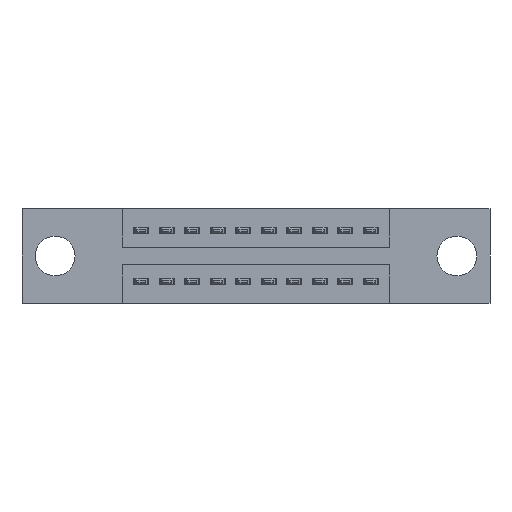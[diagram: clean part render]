
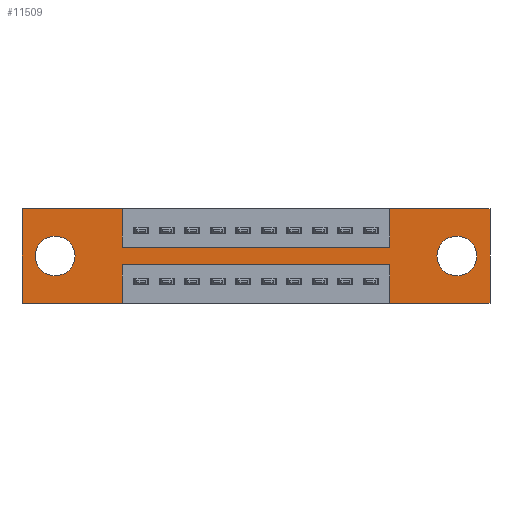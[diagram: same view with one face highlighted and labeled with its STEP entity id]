
A CAD part, front view. The second image highlights one B-rep face of the part: STEP entity #11509.
In plain terms, the highlighted planar face has unit normal (0, -1, 0).
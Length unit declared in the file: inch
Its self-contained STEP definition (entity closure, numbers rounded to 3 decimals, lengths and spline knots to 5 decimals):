
#273 = VERTEX_POINT ( 'NONE', #581 ) ;
#366 = EDGE_LOOP ( 'NONE', ( #4167, #5193, #6597, #5299, #6546, #12338, #12047, #7113, #7534, #8172, #12407, #8401 ) ) ;
#402 = DIRECTION ( 'NONE',  ( 0., 0., 1. ) ) ;
#421 = CIRCLE ( 'NONE', #2617, 0.078 ) ;
#468 = LINE ( 'NONE', #9178, #2892 ) ;
#513 = CARTESIAN_POINT ( 'NONE',  ( 0.3925, 0., -0.22 ) ) ;
#522 = VECTOR ( 'NONE', #561, 39.37008 ) ;
#561 = DIRECTION ( 'NONE',  ( 0., 0., 1. ) ) ;
#581 = CARTESIAN_POINT ( 'NONE',  ( 1.835, 0., 0. ) ) ;
#766 = DIRECTION ( 'NONE',  ( 1., 0., 0. ) ) ;
#969 = CARTESIAN_POINT ( 'NONE',  ( 0.13, 0., -0.107 ) ) ;
#1180 = EDGE_LOOP ( 'NONE', ( #1553, #4073 ) ) ;
#1264 = CARTESIAN_POINT ( 'NONE',  ( 1.835, 0., -0.37 ) ) ;
#1283 = AXIS2_PLACEMENT_3D ( 'NONE', #2928, #3809, #5951 ) ;
#1348 = DIRECTION ( 'NONE',  ( 1., 0., 0. ) ) ;
#1379 = CARTESIAN_POINT ( 'NONE',  ( 0.3925, 0., 0. ) ) ;
#1466 = VERTEX_POINT ( 'NONE', #1264 ) ;
#1487 = DIRECTION ( 'NONE',  ( 0., 0., -1. ) ) ;
#1553 = ORIENTED_EDGE ( 'NONE', *, *, #3692, .T. ) ;
#1842 = VECTOR ( 'NONE', #2558, 39.37008 ) ;
#1938 = FACE_BOUND ( 'NONE', #2115, .T. ) ;
#2027 = CARTESIAN_POINT ( 'NONE',  ( 0.3925, 0., -0.15 ) ) ;
#2050 = EDGE_CURVE ( 'NONE', #2638, #4609, #11177, .T. ) ;
#2115 = EDGE_LOOP ( 'NONE', ( #5553, #5684 ) ) ;
#2297 = CARTESIAN_POINT ( 'NONE',  ( 0., 0., -0.37 ) ) ;
#2338 = VECTOR ( 'NONE', #6648, 39.37008 ) ;
#2358 = DIRECTION ( 'NONE',  ( 0., 0., -1. ) ) ;
#2558 = DIRECTION ( 'NONE',  ( 0., 0., 1. ) ) ;
#2617 = AXIS2_PLACEMENT_3D ( 'NONE', #9967, #3362, #2358 ) ;
#2638 = VERTEX_POINT ( 'NONE', #2777 ) ;
#2651 = EDGE_CURVE ( 'NONE', #273, #1466, #9385, .T. ) ;
#2719 = DIRECTION ( 'NONE',  ( 0., 0., -1. ) ) ;
#2750 = VERTEX_POINT ( 'NONE', #2027 ) ;
#2777 = CARTESIAN_POINT ( 'NONE',  ( 1.4425, 0., -0.22 ) ) ;
#2807 = LINE ( 'NONE', #3710, #2338 ) ;
#2813 = VECTOR ( 'NONE', #9064, 39.37008 ) ;
#2825 = EDGE_CURVE ( 'NONE', #2750, #4581, #8014, .T. ) ;
#2892 = VECTOR ( 'NONE', #7827, 39.37008 ) ;
#2928 = CARTESIAN_POINT ( 'NONE',  ( 0., 0., -0.37 ) ) ;
#2982 = EDGE_CURVE ( 'NONE', #1466, #12223, #2807, .T. ) ;
#3152 = VERTEX_POINT ( 'NONE', #8782 ) ;
#3345 = CARTESIAN_POINT ( 'NONE',  ( 0.13, 0., -0.185 ) ) ;
#3356 = EDGE_CURVE ( 'NONE', #6534, #10361, #7222, .T. ) ;
#3362 = DIRECTION ( 'NONE',  ( 0., 1., 0. ) ) ;
#3375 = VERTEX_POINT ( 'NONE', #6276 ) ;
#3417 = AXIS2_PLACEMENT_3D ( 'NONE', #3345, #11262, #8382 ) ;
#3469 = LINE ( 'NONE', #6373, #8639 ) ;
#3692 = EDGE_CURVE ( 'NONE', #3375, #7938, #421, .T. ) ;
#3710 = CARTESIAN_POINT ( 'NONE',  ( 0., 0., -0.37 ) ) ;
#3809 = DIRECTION ( 'NONE',  ( 0., -1., 0. ) ) ;
#4073 = ORIENTED_EDGE ( 'NONE', *, *, #6514, .T. ) ;
#4167 = ORIENTED_EDGE ( 'NONE', *, *, #8672, .F. ) ;
#4322 = DIRECTION ( 'NONE',  ( -1., 0., 0. ) ) ;
#4442 = AXIS2_PLACEMENT_3D ( 'NONE', #8094, #7005, #1487 ) ;
#4577 = LINE ( 'NONE', #11382, #9696 ) ;
#4581 = VERTEX_POINT ( 'NONE', #10607 ) ;
#4609 = VERTEX_POINT ( 'NONE', #6147 ) ;
#4817 = CARTESIAN_POINT ( 'NONE',  ( 0.3925, 0., -0.37 ) ) ;
#5193 = ORIENTED_EDGE ( 'NONE', *, *, #2050, .F. ) ;
#5299 = ORIENTED_EDGE ( 'NONE', *, *, #2982, .F. ) ;
#5494 = CARTESIAN_POINT ( 'NONE',  ( 1.835, 0., 0. ) ) ;
#5553 = ORIENTED_EDGE ( 'NONE', *, *, #5657, .T. ) ;
#5650 = LINE ( 'NONE', #4817, #7319 ) ;
#5657 = EDGE_CURVE ( 'NONE', #9488, #3152, #8827, .T. ) ;
#5673 = EDGE_CURVE ( 'NONE', #10361, #10035, #8146, .T. ) ;
#5684 = ORIENTED_EDGE ( 'NONE', *, *, #7292, .T. ) ;
#5754 = EDGE_CURVE ( 'NONE', #10035, #2750, #3469, .T. ) ;
#5951 = DIRECTION ( 'NONE',  ( 0., 0., -1. ) ) ;
#5980 = DIRECTION ( 'NONE',  ( 0., 1., 0. ) ) ;
#5991 = CARTESIAN_POINT ( 'NONE',  ( 0.3925, 0., -0.37 ) ) ;
#6147 = CARTESIAN_POINT ( 'NONE',  ( 0.3925, 0., -0.22 ) ) ;
#6276 = CARTESIAN_POINT ( 'NONE',  ( 1.705, 0., -0.107 ) ) ;
#6373 = CARTESIAN_POINT ( 'NONE',  ( 0.3925, 0., 0. ) ) ;
#6387 = CARTESIAN_POINT ( 'NONE',  ( 1.4425, 0., -0.37 ) ) ;
#6472 = CIRCLE ( 'NONE', #9676, 0.078 ) ;
#6489 = CARTESIAN_POINT ( 'NONE',  ( 1.705, 0., -0.263 ) ) ;
#6514 = EDGE_CURVE ( 'NONE', #7938, #3375, #7465, .T. ) ;
#6534 = VERTEX_POINT ( 'NONE', #2297 ) ;
#6546 = ORIENTED_EDGE ( 'NONE', *, *, #2651, .F. ) ;
#6597 = ORIENTED_EDGE ( 'NONE', *, *, #9349, .F. ) ;
#6634 = FACE_BOUND ( 'NONE', #1180, .T. ) ;
#6648 = DIRECTION ( 'NONE',  ( -1., 0., 0. ) ) ;
#6878 = VERTEX_POINT ( 'NONE', #5991 ) ;
#7005 = DIRECTION ( 'NONE',  ( 0., 1., 0. ) ) ;
#7113 = ORIENTED_EDGE ( 'NONE', *, *, #2825, .F. ) ;
#7222 = LINE ( 'NONE', #9213, #1842 ) ;
#7292 = EDGE_CURVE ( 'NONE', #3152, #9488, #6472, .T. ) ;
#7319 = VECTOR ( 'NONE', #8556, 39.37008 ) ;
#7465 = CIRCLE ( 'NONE', #4442, 0.078 ) ;
#7485 = VERTEX_POINT ( 'NONE', #12022 ) ;
#7534 = ORIENTED_EDGE ( 'NONE', *, *, #5754, .F. ) ;
#7572 = DIRECTION ( 'NONE',  ( 0., 0., -1. ) ) ;
#7583 = LINE ( 'NONE', #11401, #12148 ) ;
#7827 = DIRECTION ( 'NONE',  ( -1., 0., 0. ) ) ;
#7938 = VERTEX_POINT ( 'NONE', #6489 ) ;
#8014 = LINE ( 'NONE', #8079, #11376 ) ;
#8079 = CARTESIAN_POINT ( 'NONE',  ( 0.3925, 0., -0.15 ) ) ;
#8094 = CARTESIAN_POINT ( 'NONE',  ( 1.705, 0., -0.185 ) ) ;
#8146 = LINE ( 'NONE', #11155, #2813 ) ;
#8172 = ORIENTED_EDGE ( 'NONE', *, *, #5673, .F. ) ;
#8308 = CARTESIAN_POINT ( 'NONE',  ( 1.4425, 0., -0.37 ) ) ;
#8382 = DIRECTION ( 'NONE',  ( 0., 0., 1. ) ) ;
#8401 = ORIENTED_EDGE ( 'NONE', *, *, #9499, .F. ) ;
#8429 = EDGE_CURVE ( 'NONE', #7485, #273, #4577, .T. ) ;
#8556 = DIRECTION ( 'NONE',  ( 0., 0., -1. ) ) ;
#8639 = VECTOR ( 'NONE', #7572, 39.37008 ) ;
#8672 = EDGE_CURVE ( 'NONE', #4609, #6878, #5650, .T. ) ;
#8782 = CARTESIAN_POINT ( 'NONE',  ( 0.13, 0., -0.263 ) ) ;
#8827 = CIRCLE ( 'NONE', #3417, 0.078 ) ;
#8965 = VECTOR ( 'NONE', #2719, 39.37008 ) ;
#9064 = DIRECTION ( 'NONE',  ( 1., 0., 0. ) ) ;
#9178 = CARTESIAN_POINT ( 'NONE',  ( 0., 0., -0.37 ) ) ;
#9213 = CARTESIAN_POINT ( 'NONE',  ( 0., 0., 0. ) ) ;
#9349 = EDGE_CURVE ( 'NONE', #12223, #2638, #11100, .T. ) ;
#9385 = LINE ( 'NONE', #5494, #8965 ) ;
#9438 = EDGE_CURVE ( 'NONE', #4581, #7485, #7583, .T. ) ;
#9488 = VERTEX_POINT ( 'NONE', #969 ) ;
#9499 = EDGE_CURVE ( 'NONE', #6878, #6534, #468, .T. ) ;
#9676 = AXIS2_PLACEMENT_3D ( 'NONE', #9942, #5980, #402 ) ;
#9696 = VECTOR ( 'NONE', #766, 39.37008 ) ;
#9942 = CARTESIAN_POINT ( 'NONE',  ( 0.13, 0., -0.185 ) ) ;
#9967 = CARTESIAN_POINT ( 'NONE',  ( 1.705, 0., -0.185 ) ) ;
#10035 = VERTEX_POINT ( 'NONE', #1379 ) ;
#10361 = VERTEX_POINT ( 'NONE', #11480 ) ;
#10456 = DIRECTION ( 'NONE',  ( 0., 0., 1. ) ) ;
#10607 = CARTESIAN_POINT ( 'NONE',  ( 1.4425, 0., -0.15 ) ) ;
#11100 = LINE ( 'NONE', #6387, #522 ) ;
#11155 = CARTESIAN_POINT ( 'NONE',  ( 0., 0., 0. ) ) ;
#11177 = LINE ( 'NONE', #513, #11585 ) ;
#11254 = PLANE ( 'NONE',  #1283 ) ;
#11262 = DIRECTION ( 'NONE',  ( 0., 1., 0. ) ) ;
#11376 = VECTOR ( 'NONE', #1348, 39.37008 ) ;
#11382 = CARTESIAN_POINT ( 'NONE',  ( 0., 0., 0. ) ) ;
#11401 = CARTESIAN_POINT ( 'NONE',  ( 1.4425, 0., 0. ) ) ;
#11480 = CARTESIAN_POINT ( 'NONE',  ( 0., 0., 0. ) ) ;
#11509 = ADVANCED_FACE ( 'NONE', ( #6634, #1938, #11609 ), #11254, .T. ) ;
#11585 = VECTOR ( 'NONE', #4322, 39.37008 ) ;
#11609 = FACE_OUTER_BOUND ( 'NONE', #366, .T. ) ;
#12022 = CARTESIAN_POINT ( 'NONE',  ( 1.4425, 0., 0. ) ) ;
#12047 = ORIENTED_EDGE ( 'NONE', *, *, #9438, .F. ) ;
#12148 = VECTOR ( 'NONE', #10456, 39.37008 ) ;
#12223 = VERTEX_POINT ( 'NONE', #8308 ) ;
#12338 = ORIENTED_EDGE ( 'NONE', *, *, #8429, .F. ) ;
#12407 = ORIENTED_EDGE ( 'NONE', *, *, #3356, .F. ) ;
